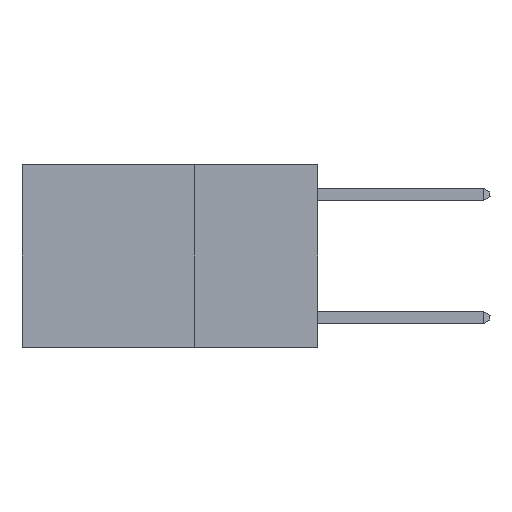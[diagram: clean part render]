
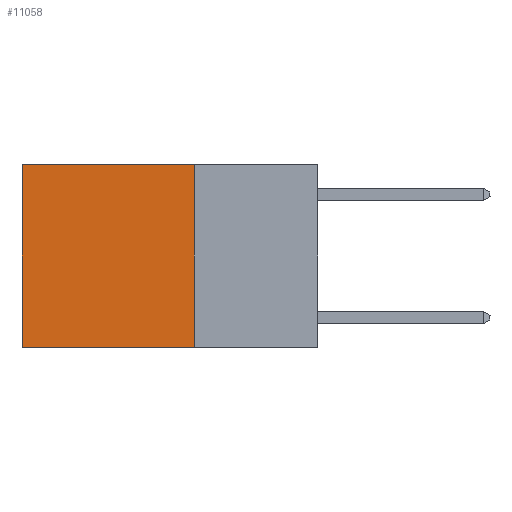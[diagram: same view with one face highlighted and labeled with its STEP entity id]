
A CAD part, left-side view. The second image highlights one B-rep face of the part: STEP entity #11058.
In plain terms, the highlighted planar face has unit normal (-1, 0, 0).
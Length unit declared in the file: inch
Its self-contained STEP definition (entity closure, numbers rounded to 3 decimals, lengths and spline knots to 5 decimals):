
#160 = LINE ( 'NONE', #10001, #10958 ) ;
#348 = CARTESIAN_POINT ( 'NONE',  ( 0.2625, 0.25, -0.37 ) ) ;
#968 = VERTEX_POINT ( 'NONE', #348 ) ;
#1095 = EDGE_LOOP ( 'NONE', ( #7621, #7350, #8949, #10096 ) ) ;
#1405 = VERTEX_POINT ( 'NONE', #6438 ) ;
#2636 = DIRECTION ( 'NONE',  ( 1., 0., 0. ) ) ;
#2763 = DIRECTION ( 'NONE',  ( 0., 1., 0. ) ) ;
#2829 = CARTESIAN_POINT ( 'NONE',  ( 0.2625, 0.25, 0. ) ) ;
#4025 = PLANE ( 'NONE',  #5131 ) ;
#4289 = EDGE_CURVE ( 'NONE', #4627, #968, #12538, .T. ) ;
#4627 = VERTEX_POINT ( 'NONE', #6759 ) ;
#4930 = FACE_OUTER_BOUND ( 'NONE', #1095, .T. ) ;
#5064 = CARTESIAN_POINT ( 'NONE',  ( 0.2625, 0.25, -0.37 ) ) ;
#5131 = AXIS2_PLACEMENT_3D ( 'NONE', #2829, #2636, #11408 ) ;
#5356 = VECTOR ( 'NONE', #2763, 39.37008 ) ;
#5461 = DIRECTION ( 'NONE',  ( 0., 1., 0. ) ) ;
#5688 = DIRECTION ( 'NONE',  ( 0., 0., -1. ) ) ;
#5731 = VECTOR ( 'NONE', #5461, 39.37008 ) ;
#5979 = DIRECTION ( 'NONE',  ( 0., 0., -1. ) ) ;
#6438 = CARTESIAN_POINT ( 'NONE',  ( 0.2625, 0.6, 0. ) ) ;
#6759 = CARTESIAN_POINT ( 'NONE',  ( 0.2625, 0.25, 0. ) ) ;
#7042 = CARTESIAN_POINT ( 'NONE',  ( 0.2625, 0.25, 0. ) ) ;
#7350 = ORIENTED_EDGE ( 'NONE', *, *, #10952, .F. ) ;
#7568 = LINE ( 'NONE', #10827, #5731 ) ;
#7606 = EDGE_CURVE ( 'NONE', #4627, #1405, #7568, .T. ) ;
#7621 = ORIENTED_EDGE ( 'NONE', *, *, #10029, .T. ) ;
#7944 = CARTESIAN_POINT ( 'NONE',  ( 0.2625, 0.6, -0.37 ) ) ;
#8949 = ORIENTED_EDGE ( 'NONE', *, *, #4289, .F. ) ;
#10001 = CARTESIAN_POINT ( 'NONE',  ( 0.2625, 0.6, 0. ) ) ;
#10029 = EDGE_CURVE ( 'NONE', #1405, #11966, #160, .T. ) ;
#10096 = ORIENTED_EDGE ( 'NONE', *, *, #7606, .T. ) ;
#10827 = CARTESIAN_POINT ( 'NONE',  ( 0.2625, 0.25, 0. ) ) ;
#10952 = EDGE_CURVE ( 'NONE', #968, #11966, #12337, .T. ) ;
#10958 = VECTOR ( 'NONE', #5688, 39.37008 ) ;
#11058 = ADVANCED_FACE ( 'NONE', ( #4930 ), #4025, .F. ) ;
#11408 = DIRECTION ( 'NONE',  ( 0., 0., -1. ) ) ;
#11966 = VERTEX_POINT ( 'NONE', #7944 ) ;
#12337 = LINE ( 'NONE', #5064, #5356 ) ;
#12538 = LINE ( 'NONE', #7042, #13583 ) ;
#13583 = VECTOR ( 'NONE', #5979, 39.37008 ) ;
